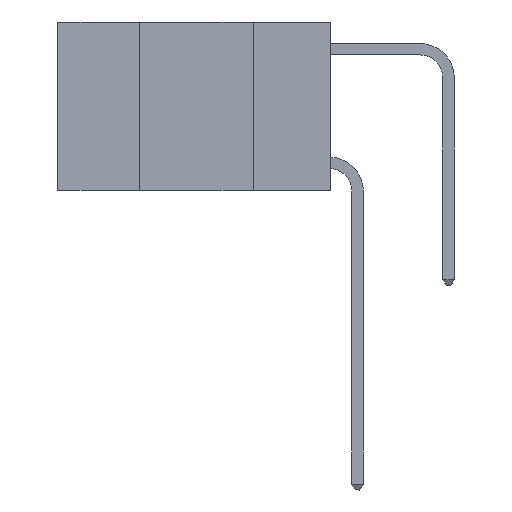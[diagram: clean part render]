
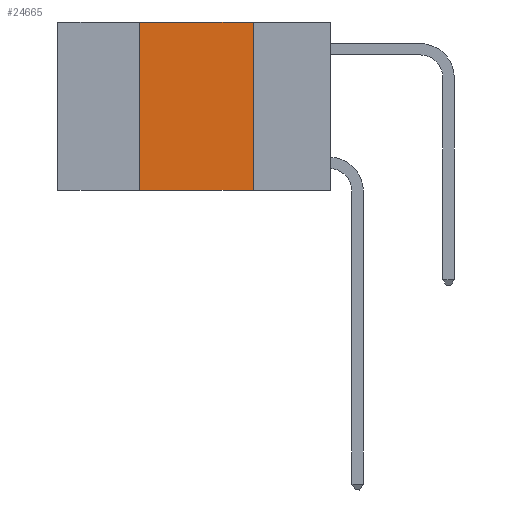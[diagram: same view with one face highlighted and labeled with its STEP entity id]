
A CAD part, left-side view. The second image highlights one B-rep face of the part: STEP entity #24665.
In plain terms, the highlighted planar face has unit normal (-1, 0, 0).
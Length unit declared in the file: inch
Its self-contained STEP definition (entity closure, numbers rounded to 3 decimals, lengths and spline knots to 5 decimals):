
#667 = ORIENTED_EDGE ( 'NONE', *, *, #27792, .T. ) ;
#939 = VECTOR ( 'NONE', #8442, 39.37008 ) ;
#2608 = VECTOR ( 'NONE', #17025, 39.37008 ) ;
#3045 = CARTESIAN_POINT ( 'NONE',  ( 0., 0.42, -0.37 ) ) ;
#3048 = ORIENTED_EDGE ( 'NONE', *, *, #20240, .F. ) ;
#3553 = EDGE_LOOP ( 'NONE', ( #23552, #21536, #3048, #667 ) ) ;
#3971 = CARTESIAN_POINT ( 'NONE',  ( 0., 0.42, 0. ) ) ;
#4256 = DIRECTION ( 'NONE',  ( 0., 0., -1. ) ) ;
#5899 = LINE ( 'NONE', #16884, #2608 ) ;
#8055 = VERTEX_POINT ( 'NONE', #13721 ) ;
#8442 = DIRECTION ( 'NONE',  ( 0., 0., 1. ) ) ;
#8576 = LINE ( 'NONE', #12445, #939 ) ;
#8964 = LINE ( 'NONE', #9260, #18738 ) ;
#9260 = CARTESIAN_POINT ( 'NONE',  ( 0., 0.17, 0. ) ) ;
#10513 = CARTESIAN_POINT ( 'NONE',  ( 0., 0.6, 0. ) ) ;
#11677 = DIRECTION ( 'NONE',  ( 0., 0., -1. ) ) ;
#12445 = CARTESIAN_POINT ( 'NONE',  ( 0., 0.42, 0. ) ) ;
#12643 = FACE_OUTER_BOUND ( 'NONE', #3553, .T. ) ;
#12803 = DIRECTION ( 'NONE',  ( 0., -1., 0. ) ) ;
#13721 = CARTESIAN_POINT ( 'NONE',  ( 0., 0.17, -0.37 ) ) ;
#14616 = AXIS2_PLACEMENT_3D ( 'NONE', #10513, #19239, #4256 ) ;
#15113 = VERTEX_POINT ( 'NONE', #16536 ) ;
#15513 = EDGE_CURVE ( 'NONE', #16610, #15113, #5899, .T. ) ;
#15777 = VERTEX_POINT ( 'NONE', #3045 ) ;
#16536 = CARTESIAN_POINT ( 'NONE',  ( 0., 0.17, 0. ) ) ;
#16610 = VERTEX_POINT ( 'NONE', #3971 ) ;
#16884 = CARTESIAN_POINT ( 'NONE',  ( 0., 0.6, 0. ) ) ;
#17025 = DIRECTION ( 'NONE',  ( 0., -1., 0. ) ) ;
#18738 = VECTOR ( 'NONE', #11677, 39.37008 ) ;
#19238 = CARTESIAN_POINT ( 'NONE',  ( 0., 0.6, -0.37 ) ) ;
#19239 = DIRECTION ( 'NONE',  ( 1., 0., 0. ) ) ;
#20240 = EDGE_CURVE ( 'NONE', #15777, #16610, #8576, .T. ) ;
#21390 = PLANE ( 'NONE',  #14616 ) ;
#21536 = ORIENTED_EDGE ( 'NONE', *, *, #15513, .F. ) ;
#22282 = VECTOR ( 'NONE', #12803, 39.37008 ) ;
#23103 = LINE ( 'NONE', #19238, #22282 ) ;
#23552 = ORIENTED_EDGE ( 'NONE', *, *, #24382, .F. ) ;
#24382 = EDGE_CURVE ( 'NONE', #15113, #8055, #8964, .T. ) ;
#24665 = ADVANCED_FACE ( 'NONE', ( #12643 ), #21390, .F. ) ;
#27792 = EDGE_CURVE ( 'NONE', #15777, #8055, #23103, .T. ) ;
